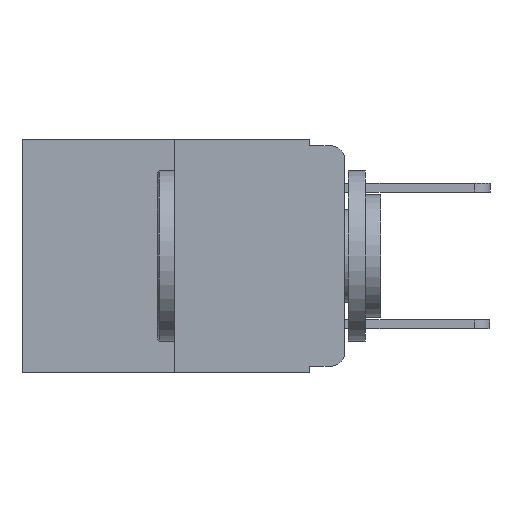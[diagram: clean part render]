
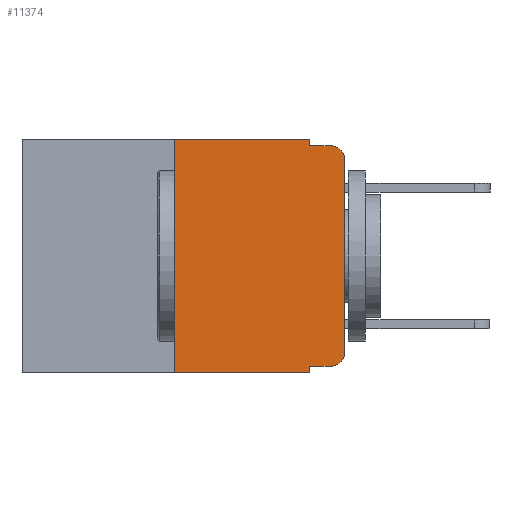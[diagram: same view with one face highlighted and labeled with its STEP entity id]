
A CAD part, left-side view. The second image highlights one B-rep face of the part: STEP entity #11374.
In plain terms, the highlighted planar face has unit normal (-1, 0, 0).
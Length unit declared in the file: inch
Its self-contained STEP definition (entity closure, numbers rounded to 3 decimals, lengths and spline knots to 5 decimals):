
#171 = CARTESIAN_POINT ( 'NONE',  ( 0., 0.25, 0. ) ) ;
#382 = DIRECTION ( 'NONE',  ( 0., -1., 0. ) ) ;
#508 = CARTESIAN_POINT ( 'NONE',  ( 0., 0.051, -0.333 ) ) ;
#805 = VECTOR ( 'NONE', #2812, 39.37008 ) ;
#859 = VECTOR ( 'NONE', #382, 39.37008 ) ;
#933 = DIRECTION ( 'NONE',  ( 0., 0., 1. ) ) ;
#1434 = CARTESIAN_POINT ( 'NONE',  ( 0., 0.02, -0.313 ) ) ;
#1521 = VERTEX_POINT ( 'NONE', #5489 ) ;
#1532 = CARTESIAN_POINT ( 'NONE',  ( 0., 0.051, -0.01 ) ) ;
#2088 = CARTESIAN_POINT ( 'NONE',  ( 0., 0.051, 0. ) ) ;
#2161 = DIRECTION ( 'NONE',  ( 0., 0., -1. ) ) ;
#2377 = VERTEX_POINT ( 'NONE', #16967 ) ;
#2408 = LINE ( 'NONE', #8864, #6074 ) ;
#2589 = DIRECTION ( 'NONE',  ( 0., -1., 0. ) ) ;
#2755 = CARTESIAN_POINT ( 'NONE',  ( 0., 0.473, -0.343 ) ) ;
#2812 = DIRECTION ( 'NONE',  ( 0., -1., 0. ) ) ;
#2865 = CARTESIAN_POINT ( 'NONE',  ( 0., 0.25, 0. ) ) ;
#2919 = EDGE_CURVE ( 'NONE', #11326, #14657, #4137, .T. ) ;
#2999 = EDGE_CURVE ( 'NONE', #14657, #2377, #3645, .T. ) ;
#3003 = DIRECTION ( 'NONE',  ( -1., 0., 0. ) ) ;
#3016 = CARTESIAN_POINT ( 'NONE',  ( 0., 0.02, -0.03 ) ) ;
#3063 = EDGE_CURVE ( 'NONE', #6720, #2377, #18027, .T. ) ;
#3153 = EDGE_CURVE ( 'NONE', #12799, #6720, #17233, .T. ) ;
#3185 = EDGE_CURVE ( 'NONE', #5067, #5749, #16847, .T. ) ;
#3225 = VERTEX_POINT ( 'NONE', #3498 ) ;
#3451 = EDGE_CURVE ( 'NONE', #3225, #6648, #2408, .T. ) ;
#3498 = CARTESIAN_POINT ( 'NONE',  ( 0., 0.051, -0.333 ) ) ;
#3533 = EDGE_CURVE ( 'NONE', #3225, #1521, #6538, .T. ) ;
#3542 = EDGE_CURVE ( 'NONE', #1521, #11326, #9198, .T. ) ;
#3645 = CIRCLE ( 'NONE', #19249, 0.02 ) ;
#3841 = DIRECTION ( 'NONE',  ( 1., 0., 0. ) ) ;
#4137 = LINE ( 'NONE', #18504, #7748 ) ;
#4214 = FACE_OUTER_BOUND ( 'NONE', #13821, .T. ) ;
#4345 = DIRECTION ( 'NONE',  ( 0., 0., 1. ) ) ;
#4949 = DIRECTION ( 'NONE',  ( 0., 0., -1. ) ) ;
#5067 = VERTEX_POINT ( 'NONE', #9881 ) ;
#5290 = DIRECTION ( 'NONE',  ( -1., 0., 0. ) ) ;
#5489 = CARTESIAN_POINT ( 'NONE',  ( 0., 0.02, -0.333 ) ) ;
#5572 = AXIS2_PLACEMENT_3D ( 'NONE', #1434, #5290, #13593 ) ;
#5749 = VERTEX_POINT ( 'NONE', #171 ) ;
#6074 = VECTOR ( 'NONE', #13610, 39.37008 ) ;
#6538 = LINE ( 'NONE', #508, #859 ) ;
#6648 = VERTEX_POINT ( 'NONE', #9655 ) ;
#6720 = VERTEX_POINT ( 'NONE', #14558 ) ;
#6844 = DIRECTION ( 'NONE',  ( 0., -1., 0. ) ) ;
#7213 = CARTESIAN_POINT ( 'NONE',  ( 0., 0.051, 0. ) ) ;
#7305 = EDGE_CURVE ( 'NONE', #5749, #12799, #10256, .T. ) ;
#7748 = VECTOR ( 'NONE', #933, 39.37008 ) ;
#8576 = ORIENTED_EDGE ( 'NONE', *, *, #2919, .T. ) ;
#8779 = ORIENTED_EDGE ( 'NONE', *, *, #2999, .T. ) ;
#8864 = CARTESIAN_POINT ( 'NONE',  ( 0., 0.051, 0. ) ) ;
#8969 = ORIENTED_EDGE ( 'NONE', *, *, #3063, .F. ) ;
#8983 = CARTESIAN_POINT ( 'NONE',  ( 0., 0.473, 0. ) ) ;
#8988 = ORIENTED_EDGE ( 'NONE', *, *, #3153, .F. ) ;
#8993 = AXIS2_PLACEMENT_3D ( 'NONE', #11603, #3841, #14576 ) ;
#9009 = ORIENTED_EDGE ( 'NONE', *, *, #7305, .F. ) ;
#9198 = CIRCLE ( 'NONE', #5572, 0.02 ) ;
#9655 = CARTESIAN_POINT ( 'NONE',  ( 0., 0.051, -0.343 ) ) ;
#9740 = ORIENTED_EDGE ( 'NONE', *, *, #3185, .F. ) ;
#9881 = CARTESIAN_POINT ( 'NONE',  ( 0., 0.25, -0.343 ) ) ;
#9891 = ORIENTED_EDGE ( 'NONE', *, *, #11567, .T. ) ;
#9895 = ORIENTED_EDGE ( 'NONE', *, *, #3451, .F. ) ;
#9940 = ORIENTED_EDGE ( 'NONE', *, *, #3533, .T. ) ;
#10256 = LINE ( 'NONE', #8983, #13323 ) ;
#10469 = VECTOR ( 'NONE', #2589, 39.37008 ) ;
#10777 = ORIENTED_EDGE ( 'NONE', *, *, #3542, .T. ) ;
#11326 = VERTEX_POINT ( 'NONE', #12631 ) ;
#11374 = ADVANCED_FACE ( 'NONE', ( #4214 ), #13078, .F. ) ;
#11567 = EDGE_CURVE ( 'NONE', #5067, #6648, #13221, .T. ) ;
#11603 = CARTESIAN_POINT ( 'NONE',  ( 0., 0.473, 0. ) ) ;
#12631 = CARTESIAN_POINT ( 'NONE',  ( 0., 0., -0.313 ) ) ;
#12799 = VERTEX_POINT ( 'NONE', #7213 ) ;
#13056 = VECTOR ( 'NONE', #4345, 39.37008 ) ;
#13078 = PLANE ( 'NONE',  #8993 ) ;
#13221 = LINE ( 'NONE', #2755, #805 ) ;
#13323 = VECTOR ( 'NONE', #6844, 39.37008 ) ;
#13515 = VECTOR ( 'NONE', #2161, 39.37008 ) ;
#13593 = DIRECTION ( 'NONE',  ( 0., 0., -1. ) ) ;
#13610 = DIRECTION ( 'NONE',  ( 0., 0., -1. ) ) ;
#13821 = EDGE_LOOP ( 'NONE', ( #8576, #8779, #8969, #8988, #9009, #9740, #9891, #9895, #9940, #10777 ) ) ;
#14558 = CARTESIAN_POINT ( 'NONE',  ( 0., 0.051, -0.01 ) ) ;
#14576 = DIRECTION ( 'NONE',  ( 0., 0., -1. ) ) ;
#14657 = VERTEX_POINT ( 'NONE', #17446 ) ;
#16847 = LINE ( 'NONE', #2865, #13056 ) ;
#16967 = CARTESIAN_POINT ( 'NONE',  ( 0., 0.02, -0.01 ) ) ;
#17233 = LINE ( 'NONE', #2088, #13515 ) ;
#17446 = CARTESIAN_POINT ( 'NONE',  ( 0., 0., -0.03 ) ) ;
#18027 = LINE ( 'NONE', #1532, #10469 ) ;
#18504 = CARTESIAN_POINT ( 'NONE',  ( 0., 0., 0. ) ) ;
#19249 = AXIS2_PLACEMENT_3D ( 'NONE', #3016, #3003, #4949 ) ;
